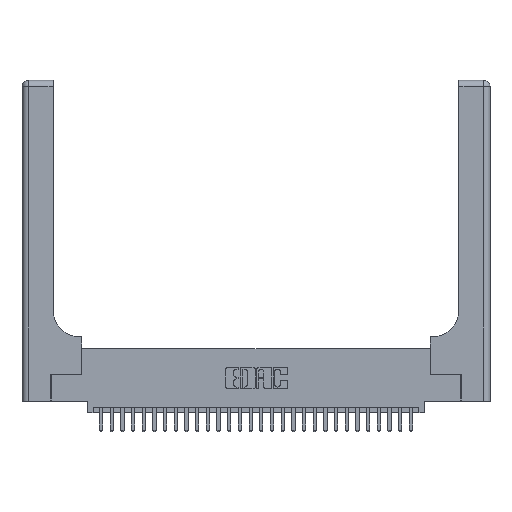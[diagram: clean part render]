
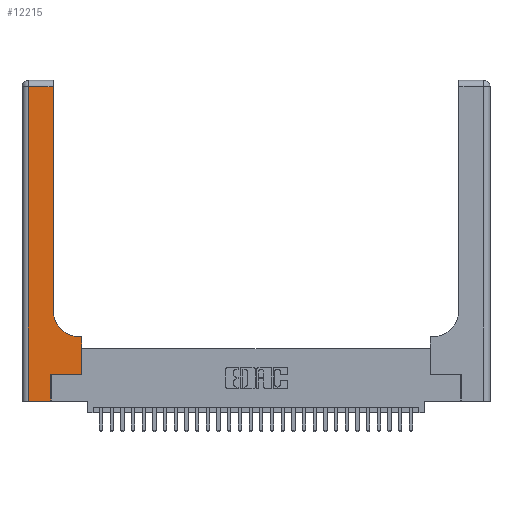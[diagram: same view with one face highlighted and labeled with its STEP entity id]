
A CAD part, top view. The second image highlights one B-rep face of the part: STEP entity #12215.
In plain terms, the highlighted planar face has unit normal (0, 0, 1).
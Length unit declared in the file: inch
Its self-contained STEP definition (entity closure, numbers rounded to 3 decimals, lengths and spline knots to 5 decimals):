
#1089 = LINE ( 'NONE', #10975, #18610 ) ;
#1550 = VERTEX_POINT ( 'NONE', #15783 ) ;
#1712 = VERTEX_POINT ( 'NONE', #18857 ) ;
#2015 = CARTESIAN_POINT ( 'NONE',  ( 0.269, 0., 0.37 ) ) ;
#2290 = ORIENTED_EDGE ( 'NONE', *, *, #8920, .T. ) ;
#2685 = VERTEX_POINT ( 'NONE', #14997 ) ;
#3027 = ORIENTED_EDGE ( 'NONE', *, *, #23902, .T. ) ;
#3368 = CIRCLE ( 'NONE', #25203, 0.25 ) ;
#3517 = CARTESIAN_POINT ( 'NONE',  ( 0., 2.94, 0.37 ) ) ;
#4154 = EDGE_CURVE ( 'NONE', #28602, #14983, #1089, .T. ) ;
#4882 = PLANE ( 'NONE',  #18434 ) ;
#5575 = VERTEX_POINT ( 'NONE', #25287 ) ;
#5711 = EDGE_CURVE ( 'NONE', #22155, #5575, #16668, .T. ) ;
#6859 = DIRECTION ( 'NONE',  ( 0., 1., 0. ) ) ;
#7725 = LINE ( 'NONE', #27773, #25113 ) ;
#8504 = LINE ( 'NONE', #22304, #26617 ) ;
#8816 = ORIENTED_EDGE ( 'NONE', *, *, #16006, .T. ) ;
#8906 = DIRECTION ( 'NONE',  ( 1., 0., 0. ) ) ;
#8920 = EDGE_CURVE ( 'NONE', #5575, #27440, #25529, .T. ) ;
#9612 = EDGE_CURVE ( 'NONE', #1712, #22155, #7725, .T. ) ;
#9683 = DIRECTION ( 'NONE',  ( -1., 0., 0. ) ) ;
#10039 = VECTOR ( 'NONE', #27995, 39.37008 ) ;
#10343 = VECTOR ( 'NONE', #6859, 39.37008 ) ;
#10501 = DIRECTION ( 'NONE',  ( 0., -1., 0. ) ) ;
#10708 = DIRECTION ( 'NONE',  ( -1., 0., 0. ) ) ;
#10975 = CARTESIAN_POINT ( 'NONE',  ( 0.2915, 3., 0.37 ) ) ;
#11208 = DIRECTION ( 'NONE',  ( 1., 0., 0. ) ) ;
#11311 = CARTESIAN_POINT ( 'NONE',  ( 0.269, 0.25, 0.37 ) ) ;
#11514 = CARTESIAN_POINT ( 'NONE',  ( 0.5585, 0.25, 0.37 ) ) ;
#12008 = CARTESIAN_POINT ( 'NONE',  ( 0.5415, 0.85, 0.37 ) ) ;
#12209 = VECTOR ( 'NONE', #11208, 39.37008 ) ;
#12215 = ADVANCED_FACE ( 'NONE', ( #24996 ), #4882, .F. ) ;
#13830 = EDGE_CURVE ( 'NONE', #14983, #1550, #21340, .T. ) ;
#14411 = DIRECTION ( 'NONE',  ( 1., 0., 0. ) ) ;
#14983 = VERTEX_POINT ( 'NONE', #15199 ) ;
#14997 = CARTESIAN_POINT ( 'NONE',  ( 0.5585, 0.6, 0.37 ) ) ;
#15199 = CARTESIAN_POINT ( 'NONE',  ( 0.2915, 2.94, 0.37 ) ) ;
#15783 = CARTESIAN_POINT ( 'NONE',  ( 0.06, 2.94, 0.37 ) ) ;
#15974 = EDGE_LOOP ( 'NONE', ( #21920, #16221, #3027, #23461, #16827, #2290, #19135, #28707, #8816 ) ) ;
#16006 = EDGE_CURVE ( 'NONE', #22022, #28602, #3368, .T. ) ;
#16221 = ORIENTED_EDGE ( 'NONE', *, *, #13830, .T. ) ;
#16494 = CARTESIAN_POINT ( 'NONE',  ( 0.5585, 0.25, 0.37 ) ) ;
#16515 = DIRECTION ( 'NONE',  ( -1., 0., 0. ) ) ;
#16668 = LINE ( 'NONE', #2015, #10343 ) ;
#16827 = ORIENTED_EDGE ( 'NONE', *, *, #5711, .T. ) ;
#17237 = VECTOR ( 'NONE', #16515, 39.37008 ) ;
#18434 = AXIS2_PLACEMENT_3D ( 'NONE', #21464, #23831, #9683 ) ;
#18610 = VECTOR ( 'NONE', #29769, 39.37008 ) ;
#18857 = CARTESIAN_POINT ( 'NONE',  ( 0.06, 0., 0.37 ) ) ;
#19135 = ORIENTED_EDGE ( 'NONE', *, *, #27347, .T. ) ;
#20118 = CARTESIAN_POINT ( 'NONE',  ( 0.269, 0., 0.37 ) ) ;
#20545 = EDGE_CURVE ( 'NONE', #2685, #22022, #23519, .T. ) ;
#21340 = LINE ( 'NONE', #3517, #26842 ) ;
#21464 = CARTESIAN_POINT ( 'NONE',  ( 0., 3., 0.37 ) ) ;
#21920 = ORIENTED_EDGE ( 'NONE', *, *, #4154, .T. ) ;
#22022 = VERTEX_POINT ( 'NONE', #26709 ) ;
#22155 = VERTEX_POINT ( 'NONE', #20118 ) ;
#22304 = CARTESIAN_POINT ( 'NONE',  ( 0.06, 3., 0.37 ) ) ;
#23461 = ORIENTED_EDGE ( 'NONE', *, *, #9612, .T. ) ;
#23519 = LINE ( 'NONE', #25903, #17237 ) ;
#23831 = DIRECTION ( 'NONE',  ( 0., 0., -1. ) ) ;
#23902 = EDGE_CURVE ( 'NONE', #1550, #1712, #8504, .T. ) ;
#24996 = FACE_OUTER_BOUND ( 'NONE', #15974, .T. ) ;
#25113 = VECTOR ( 'NONE', #8906, 39.37008 ) ;
#25203 = AXIS2_PLACEMENT_3D ( 'NONE', #12008, #28467, #14411 ) ;
#25287 = CARTESIAN_POINT ( 'NONE',  ( 0.269, 0.25, 0.37 ) ) ;
#25529 = LINE ( 'NONE', #11311, #12209 ) ;
#25812 = CARTESIAN_POINT ( 'NONE',  ( 0.2915, 0.85, 0.37 ) ) ;
#25903 = CARTESIAN_POINT ( 'NONE',  ( 0.2915, 0.6, 0.37 ) ) ;
#26617 = VECTOR ( 'NONE', #10501, 39.37008 ) ;
#26709 = CARTESIAN_POINT ( 'NONE',  ( 0.5415, 0.6, 0.37 ) ) ;
#26842 = VECTOR ( 'NONE', #10708, 39.37008 ) ;
#27347 = EDGE_CURVE ( 'NONE', #27440, #2685, #27370, .T. ) ;
#27370 = LINE ( 'NONE', #11514, #10039 ) ;
#27440 = VERTEX_POINT ( 'NONE', #16494 ) ;
#27773 = CARTESIAN_POINT ( 'NONE',  ( 0., 0., 0.37 ) ) ;
#27995 = DIRECTION ( 'NONE',  ( 0., 1., 0. ) ) ;
#28467 = DIRECTION ( 'NONE',  ( 0., 0., -1. ) ) ;
#28602 = VERTEX_POINT ( 'NONE', #25812 ) ;
#28707 = ORIENTED_EDGE ( 'NONE', *, *, #20545, .T. ) ;
#29769 = DIRECTION ( 'NONE',  ( 0., 1., 0. ) ) ;
